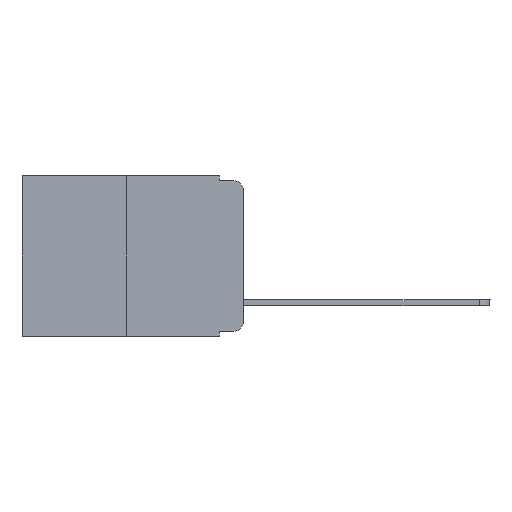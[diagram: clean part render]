
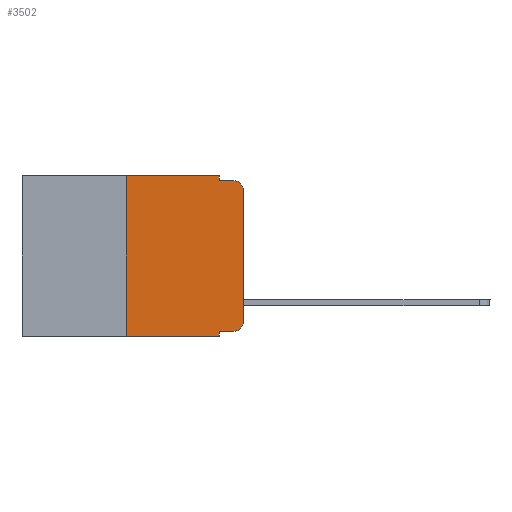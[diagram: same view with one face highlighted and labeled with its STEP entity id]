
A CAD part, left-side view. The second image highlights one B-rep face of the part: STEP entity #3502.
In plain terms, the highlighted planar face has unit normal (-1, 0, 0).
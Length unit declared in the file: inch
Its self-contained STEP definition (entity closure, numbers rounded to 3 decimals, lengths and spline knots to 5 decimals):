
#947 = DIRECTION ( 'NONE',  ( 0., 0., -1. ) ) ;
#1323 = CARTESIAN_POINT ( 'NONE',  ( 0., 0.051, -0.343 ) ) ;
#1344 = DIRECTION ( 'NONE',  ( 0., -1., 0. ) ) ;
#1907 = DIRECTION ( 'NONE',  ( 0., 0., -1. ) ) ;
#1991 = DIRECTION ( 'NONE',  ( 1., 0., 0. ) ) ;
#2324 = ORIENTED_EDGE ( 'NONE', *, *, #5090, .T. ) ;
#2448 = FACE_OUTER_BOUND ( 'NONE', #16855, .T. ) ;
#2729 = VERTEX_POINT ( 'NONE', #14893 ) ;
#3289 = LINE ( 'NONE', #3952, #12040 ) ;
#3301 = DIRECTION ( 'NONE',  ( 0., 0., -1. ) ) ;
#3472 = EDGE_CURVE ( 'NONE', #15392, #2729, #3289, .T. ) ;
#3502 = ADVANCED_FACE ( 'NONE', ( #2448 ), #18060, .F. ) ;
#3571 = CARTESIAN_POINT ( 'NONE',  ( 0., 0.051, 0. ) ) ;
#3952 = CARTESIAN_POINT ( 'NONE',  ( 0., 0., 0. ) ) ;
#4174 = DIRECTION ( 'NONE',  ( 0., 0., -1. ) ) ;
#4472 = CARTESIAN_POINT ( 'NONE',  ( 0., 0.25, 0. ) ) ;
#4663 = VECTOR ( 'NONE', #7958, 39.37008 ) ;
#5090 = EDGE_CURVE ( 'NONE', #2729, #7323, #6579, .T. ) ;
#5342 = VERTEX_POINT ( 'NONE', #21848 ) ;
#5434 = AXIS2_PLACEMENT_3D ( 'NONE', #11978, #19193, #947 ) ;
#5594 = DIRECTION ( 'NONE',  ( 0., 0., 1. ) ) ;
#6361 = ORIENTED_EDGE ( 'NONE', *, *, #13797, .T. ) ;
#6419 = VERTEX_POINT ( 'NONE', #13340 ) ;
#6579 = CIRCLE ( 'NONE', #8816, 0.02 ) ;
#6774 = VECTOR ( 'NONE', #7994, 39.37008 ) ;
#6998 = ORIENTED_EDGE ( 'NONE', *, *, #13106, .T. ) ;
#7036 = CIRCLE ( 'NONE', #5434, 0.02 ) ;
#7323 = VERTEX_POINT ( 'NONE', #19416 ) ;
#7818 = VERTEX_POINT ( 'NONE', #16097 ) ;
#7958 = DIRECTION ( 'NONE',  ( 0., -1., 0. ) ) ;
#7994 = DIRECTION ( 'NONE',  ( 0., 0., 1. ) ) ;
#8002 = DIRECTION ( 'NONE',  ( 0., -1., 0. ) ) ;
#8816 = AXIS2_PLACEMENT_3D ( 'NONE', #17429, #14066, #3301 ) ;
#9087 = CARTESIAN_POINT ( 'NONE',  ( 0., 0.473, 0. ) ) ;
#9353 = VECTOR ( 'NONE', #1344, 39.37008 ) ;
#9534 = VECTOR ( 'NONE', #4174, 39.37008 ) ;
#9632 = VERTEX_POINT ( 'NONE', #3571 ) ;
#10029 = EDGE_CURVE ( 'NONE', #5342, #18639, #11878, .T. ) ;
#10190 = VERTEX_POINT ( 'NONE', #10652 ) ;
#10566 = EDGE_CURVE ( 'NONE', #5342, #7818, #20489, .T. ) ;
#10652 = CARTESIAN_POINT ( 'NONE',  ( 0., 0.051, -0.01 ) ) ;
#10678 = CARTESIAN_POINT ( 'NONE',  ( 0., 0.02, -0.333 ) ) ;
#11529 = CARTESIAN_POINT ( 'NONE',  ( 0., 0.051, -0.333 ) ) ;
#11693 = CARTESIAN_POINT ( 'NONE',  ( 0., 0., -0.313 ) ) ;
#11786 = EDGE_CURVE ( 'NONE', #9632, #10190, #18435, .T. ) ;
#11792 = VECTOR ( 'NONE', #17822, 39.37008 ) ;
#11878 = LINE ( 'NONE', #22796, #9353 ) ;
#11940 = LINE ( 'NONE', #18683, #22528 ) ;
#11978 = CARTESIAN_POINT ( 'NONE',  ( 0., 0.02, -0.313 ) ) ;
#12040 = VECTOR ( 'NONE', #5594, 39.37008 ) ;
#12388 = AXIS2_PLACEMENT_3D ( 'NONE', #9087, #1991, #1907 ) ;
#12704 = ORIENTED_EDGE ( 'NONE', *, *, #10029, .T. ) ;
#13106 = EDGE_CURVE ( 'NONE', #6419, #20625, #18941, .T. ) ;
#13340 = CARTESIAN_POINT ( 'NONE',  ( 0., 0.051, -0.333 ) ) ;
#13662 = ORIENTED_EDGE ( 'NONE', *, *, #17071, .F. ) ;
#13797 = EDGE_CURVE ( 'NONE', #20625, #15392, #7036, .T. ) ;
#14066 = DIRECTION ( 'NONE',  ( -1., 0., 0. ) ) ;
#14377 = EDGE_CURVE ( 'NONE', #10190, #7323, #18741, .T. ) ;
#14403 = CARTESIAN_POINT ( 'NONE',  ( 0., 0.051, -0.01 ) ) ;
#14681 = EDGE_CURVE ( 'NONE', #7818, #9632, #17370, .T. ) ;
#14868 = CARTESIAN_POINT ( 'NONE',  ( 0., 0.051, 0. ) ) ;
#14893 = CARTESIAN_POINT ( 'NONE',  ( 0., 0., -0.03 ) ) ;
#15392 = VERTEX_POINT ( 'NONE', #11693 ) ;
#16097 = CARTESIAN_POINT ( 'NONE',  ( 0., 0.25, 0. ) ) ;
#16103 = ORIENTED_EDGE ( 'NONE', *, *, #14681, .F. ) ;
#16293 = ORIENTED_EDGE ( 'NONE', *, *, #3472, .T. ) ;
#16855 = EDGE_LOOP ( 'NONE', ( #16293, #2324, #19230, #19605, #16103, #19978, #12704, #13662, #6998, #6361 ) ) ;
#16872 = CARTESIAN_POINT ( 'NONE',  ( 0., 0.473, 0. ) ) ;
#17071 = EDGE_CURVE ( 'NONE', #6419, #18639, #11940, .T. ) ;
#17370 = LINE ( 'NONE', #16872, #23230 ) ;
#17429 = CARTESIAN_POINT ( 'NONE',  ( 0., 0.02, -0.03 ) ) ;
#17822 = DIRECTION ( 'NONE',  ( 0., -1., 0. ) ) ;
#18060 = PLANE ( 'NONE',  #12388 ) ;
#18435 = LINE ( 'NONE', #14868, #9534 ) ;
#18639 = VERTEX_POINT ( 'NONE', #1323 ) ;
#18683 = CARTESIAN_POINT ( 'NONE',  ( 0., 0.051, 0. ) ) ;
#18741 = LINE ( 'NONE', #14403, #11792 ) ;
#18941 = LINE ( 'NONE', #11529, #4663 ) ;
#19193 = DIRECTION ( 'NONE',  ( -1., 0., 0. ) ) ;
#19230 = ORIENTED_EDGE ( 'NONE', *, *, #14377, .F. ) ;
#19416 = CARTESIAN_POINT ( 'NONE',  ( 0., 0.02, -0.01 ) ) ;
#19605 = ORIENTED_EDGE ( 'NONE', *, *, #11786, .F. ) ;
#19978 = ORIENTED_EDGE ( 'NONE', *, *, #10566, .F. ) ;
#20489 = LINE ( 'NONE', #4472, #6774 ) ;
#20493 = DIRECTION ( 'NONE',  ( 0., 0., -1. ) ) ;
#20625 = VERTEX_POINT ( 'NONE', #10678 ) ;
#21848 = CARTESIAN_POINT ( 'NONE',  ( 0., 0.25, -0.343 ) ) ;
#22528 = VECTOR ( 'NONE', #20493, 39.37008 ) ;
#22796 = CARTESIAN_POINT ( 'NONE',  ( 0., 0.473, -0.343 ) ) ;
#23230 = VECTOR ( 'NONE', #8002, 39.37008 ) ;
